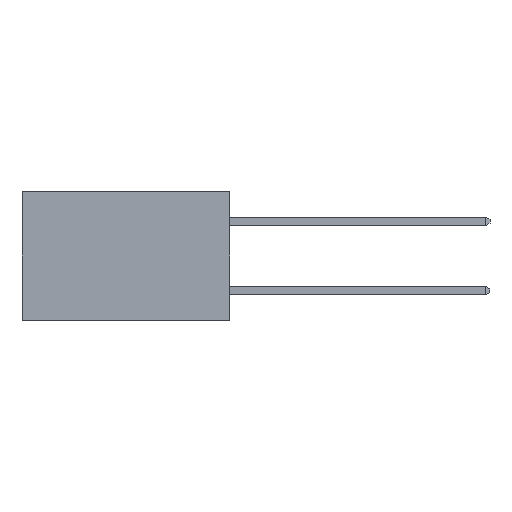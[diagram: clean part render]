
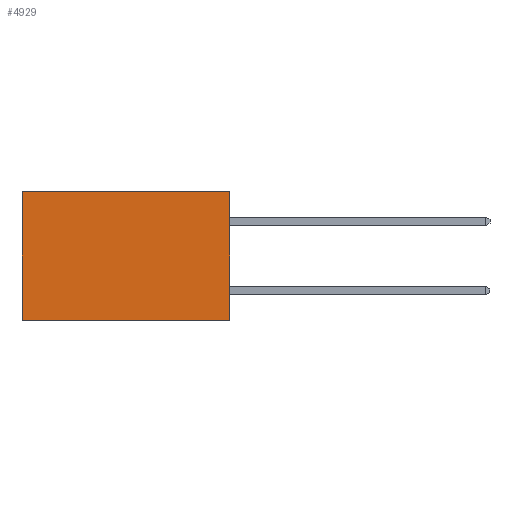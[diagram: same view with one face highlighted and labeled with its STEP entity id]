
A CAD part, left-side view. The second image highlights one B-rep face of the part: STEP entity #4929.
In plain terms, the highlighted planar face has unit normal (-1, 0, 0).
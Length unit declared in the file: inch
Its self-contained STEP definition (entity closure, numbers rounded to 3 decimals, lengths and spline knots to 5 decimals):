
#91 = VECTOR ( 'NONE', #5390, 39.37008 ) ;
#293 = EDGE_CURVE ( 'NONE', #8215, #7147, #6028, .T. ) ;
#345 = VECTOR ( 'NONE', #7522, 39.37008 ) ;
#653 = CARTESIAN_POINT ( 'NONE',  ( 0.298, 0., 0. ) ) ;
#1116 = ORIENTED_EDGE ( 'NONE', *, *, #293, .T. ) ;
#1163 = DIRECTION ( 'NONE',  ( 0., 0., -1. ) ) ;
#1185 = DIRECTION ( 'NONE',  ( 1., 0., 0. ) ) ;
#1247 = CARTESIAN_POINT ( 'NONE',  ( 0.298, 0., 0. ) ) ;
#1278 = ORIENTED_EDGE ( 'NONE', *, *, #8090, .F. ) ;
#1397 = EDGE_LOOP ( 'NONE', ( #1116, #1278, #1492, #1634 ) ) ;
#1467 = LINE ( 'NONE', #1703, #10728 ) ;
#1492 = ORIENTED_EDGE ( 'NONE', *, *, #5766, .F. ) ;
#1634 = ORIENTED_EDGE ( 'NONE', *, *, #1721, .T. ) ;
#1703 = CARTESIAN_POINT ( 'NONE',  ( 0.298, 0., 0. ) ) ;
#1718 = VERTEX_POINT ( 'NONE', #4033 ) ;
#1721 = EDGE_CURVE ( 'NONE', #2118, #8215, #1467, .T. ) ;
#2118 = VERTEX_POINT ( 'NONE', #653 ) ;
#2633 = AXIS2_PLACEMENT_3D ( 'NONE', #1247, #1185, #1163 ) ;
#2880 = LINE ( 'NONE', #7833, #345 ) ;
#3090 = PLANE ( 'NONE',  #2633 ) ;
#3404 = CARTESIAN_POINT ( 'NONE',  ( 0.298, 0.6, 0. ) ) ;
#4033 = CARTESIAN_POINT ( 'NONE',  ( 0.298, 0., -0.37 ) ) ;
#4664 = CARTESIAN_POINT ( 'NONE',  ( 0.298, 0.6, 0. ) ) ;
#4929 = ADVANCED_FACE ( 'NONE', ( #10040 ), #3090, .F. ) ;
#5077 = DIRECTION ( 'NONE',  ( 0., 1., 0. ) ) ;
#5390 = DIRECTION ( 'NONE',  ( 0., 1., 0. ) ) ;
#5415 = CARTESIAN_POINT ( 'NONE',  ( 0.298, 0., -0.37 ) ) ;
#5766 = EDGE_CURVE ( 'NONE', #2118, #1718, #2880, .T. ) ;
#6028 = LINE ( 'NONE', #3404, #10366 ) ;
#7147 = VERTEX_POINT ( 'NONE', #10860 ) ;
#7522 = DIRECTION ( 'NONE',  ( 0., 0., -1. ) ) ;
#7833 = CARTESIAN_POINT ( 'NONE',  ( 0.298, 0., 0. ) ) ;
#8090 = EDGE_CURVE ( 'NONE', #1718, #7147, #9541, .T. ) ;
#8215 = VERTEX_POINT ( 'NONE', #4664 ) ;
#9541 = LINE ( 'NONE', #5415, #91 ) ;
#10040 = FACE_OUTER_BOUND ( 'NONE', #1397, .T. ) ;
#10252 = DIRECTION ( 'NONE',  ( 0., 0., -1. ) ) ;
#10366 = VECTOR ( 'NONE', #10252, 39.37008 ) ;
#10728 = VECTOR ( 'NONE', #5077, 39.37008 ) ;
#10860 = CARTESIAN_POINT ( 'NONE',  ( 0.298, 0.6, -0.37 ) ) ;
